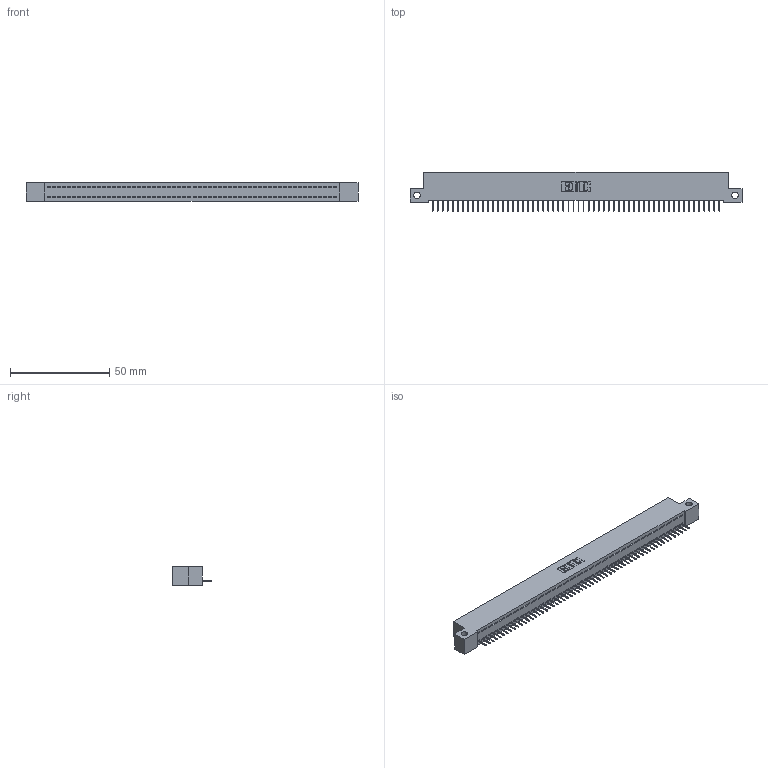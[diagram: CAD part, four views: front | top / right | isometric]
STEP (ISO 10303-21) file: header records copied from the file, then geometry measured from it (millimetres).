
FILE_DESCRIPTION (( 'STEP AP203' ), '1' );
FILE_NAME ('342-058-524-112.STEP', '2019-10-03T12:36:40', ( '' ), ( '' ), 'SwSTEP 2.0', 'SolidWorks 2016', '' );
FILE_SCHEMA (( 'CONFIG_CONTROL_DESIGN' ));
Length unit declared in the file: inch
Products named in the file (3): 345-292-001_345-293-124; 342-058-524-112; 342 Part_Side Mount
Assembly tree (59 placements, depth 2):
  342-058-524-112
    342 Part_Side Mount
    345-292-001_345-293-124  x58
Bounding box: 167.64 x 19.69 x 9.4 mm (x, y, z)
Volume: 14454.6 mm3; surface area: 20649.9 mm2
Topology: 59 solids, 59 shells, 3706 faces, 10739 edges, 6926 vertices
Faces by surface type: plane 2850, cylinder 856
Entity records: 33333 total; most frequent: CARTESIAN_POINT 5752, ORIENTED_EDGE 5746, DIRECTION 4821, EDGE_CURVE 2873, LINE 2749, VECTOR 2749, VERTEX_POINT 1910, AXIS2_PLACEMENT_3D 1036
